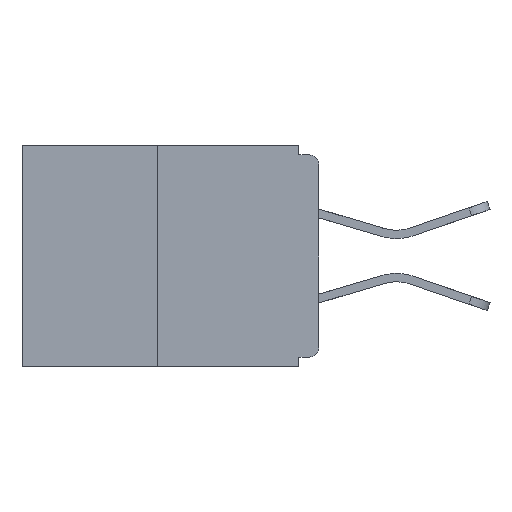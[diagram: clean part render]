
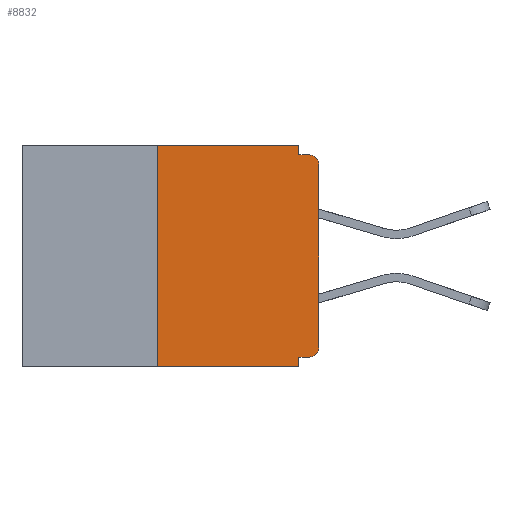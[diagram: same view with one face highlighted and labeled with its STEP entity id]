
A CAD part, left-side view. The second image highlights one B-rep face of the part: STEP entity #8832.
In plain terms, the highlighted planar face has unit normal (-1, 0, 0).
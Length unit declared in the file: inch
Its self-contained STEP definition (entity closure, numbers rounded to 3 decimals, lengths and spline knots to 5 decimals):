
#118 = ORIENTED_EDGE ( 'NONE', *, *, #2227, .F. ) ;
#169 = VERTEX_POINT ( 'NONE', #3268 ) ;
#374 = CARTESIAN_POINT ( 'NONE',  ( 0., 0.031, 0. ) ) ;
#448 = DIRECTION ( 'NONE',  ( 0., -1., 0. ) ) ;
#489 = CARTESIAN_POINT ( 'NONE',  ( 0., 0.46, 0. ) ) ;
#515 = CARTESIAN_POINT ( 'NONE',  ( 0., 0.015, -0.328 ) ) ;
#697 = FACE_OUTER_BOUND ( 'NONE', #9683, .T. ) ;
#770 = CARTESIAN_POINT ( 'NONE',  ( 0., 0., -0.03 ) ) ;
#947 = ORIENTED_EDGE ( 'NONE', *, *, #1244, .T. ) ;
#956 = AXIS2_PLACEMENT_3D ( 'NONE', #5543, #6500, #9940 ) ;
#1126 = CARTESIAN_POINT ( 'NONE',  ( 0., 0., -0.328 ) ) ;
#1204 = DIRECTION ( 'NONE',  ( 0., 1., 0. ) ) ;
#1244 = EDGE_CURVE ( 'NONE', #8211, #8496, #11496, .T. ) ;
#1271 = DIRECTION ( 'NONE',  ( 0., 0., -1. ) ) ;
#1419 = ORIENTED_EDGE ( 'NONE', *, *, #4956, .F. ) ;
#1483 = EDGE_CURVE ( 'NONE', #9737, #9106, #4185, .T. ) ;
#2227 = EDGE_CURVE ( 'NONE', #6264, #7091, #10370, .T. ) ;
#2407 = DIRECTION ( 'NONE',  ( 0., 0., -1. ) ) ;
#2658 = LINE ( 'NONE', #1126, #7680 ) ;
#2899 = CARTESIAN_POINT ( 'NONE',  ( 0., 0., 0. ) ) ;
#2945 = CARTESIAN_POINT ( 'NONE',  ( 0., 0.015, -0.015 ) ) ;
#3024 = VECTOR ( 'NONE', #1271, 39.37008 ) ;
#3134 = VECTOR ( 'NONE', #3990, 39.37008 ) ;
#3176 = AXIS2_PLACEMENT_3D ( 'NONE', #8057, #5354, #6136 ) ;
#3268 = CARTESIAN_POINT ( 'NONE',  ( 0., 0.031, -0.015 ) ) ;
#3499 = DIRECTION ( 'NONE',  ( 0., 0., -1. ) ) ;
#3785 = VECTOR ( 'NONE', #9099, 39.37008 ) ;
#3952 = LINE ( 'NONE', #489, #9489 ) ;
#3979 = CARTESIAN_POINT ( 'NONE',  ( 0., 0.25, 0. ) ) ;
#3990 = DIRECTION ( 'NONE',  ( 0., -1., 0. ) ) ;
#4185 = CIRCLE ( 'NONE', #3176, 0.015 ) ;
#4748 = CARTESIAN_POINT ( 'NONE',  ( 0., 0., -0.015 ) ) ;
#4904 = ORIENTED_EDGE ( 'NONE', *, *, #7840, .F. ) ;
#4956 = EDGE_CURVE ( 'NONE', #10288, #169, #10621, .T. ) ;
#4982 = CARTESIAN_POINT ( 'NONE',  ( 0., 0.46, -0.343 ) ) ;
#5097 = DIRECTION ( 'NONE',  ( -1., 0., 0. ) ) ;
#5354 = DIRECTION ( 'NONE',  ( -1., 0., 0. ) ) ;
#5543 = CARTESIAN_POINT ( 'NONE',  ( 0., 0.46, 0. ) ) ;
#5566 = CARTESIAN_POINT ( 'NONE',  ( 0., 0.031, 0. ) ) ;
#6071 = DIRECTION ( 'NONE',  ( 0., 0., 1. ) ) ;
#6089 = VECTOR ( 'NONE', #6071, 39.37008 ) ;
#6136 = DIRECTION ( 'NONE',  ( 0., 0., -1. ) ) ;
#6165 = EDGE_CURVE ( 'NONE', #169, #9106, #8672, .T. ) ;
#6255 = CARTESIAN_POINT ( 'NONE',  ( 0., 0.031, -0.343 ) ) ;
#6264 = VERTEX_POINT ( 'NONE', #6906 ) ;
#6500 = DIRECTION ( 'NONE',  ( 1., 0., 0. ) ) ;
#6684 = CARTESIAN_POINT ( 'NONE',  ( 0., 0.015, -0.313 ) ) ;
#6906 = CARTESIAN_POINT ( 'NONE',  ( 0., 0.25, -0.343 ) ) ;
#7042 = CARTESIAN_POINT ( 'NONE',  ( 0., 0.25, 0. ) ) ;
#7090 = LINE ( 'NONE', #6255, #9736 ) ;
#7091 = VERTEX_POINT ( 'NONE', #3979 ) ;
#7163 = CARTESIAN_POINT ( 'NONE',  ( 0., 0.031, -0.343 ) ) ;
#7203 = ORIENTED_EDGE ( 'NONE', *, *, #1483, .T. ) ;
#7227 = ORIENTED_EDGE ( 'NONE', *, *, #6165, .F. ) ;
#7264 = ORIENTED_EDGE ( 'NONE', *, *, #7390, .T. ) ;
#7390 = EDGE_CURVE ( 'NONE', #8496, #9737, #11139, .T. ) ;
#7397 = EDGE_CURVE ( 'NONE', #8211, #7767, #2658, .T. ) ;
#7423 = CARTESIAN_POINT ( 'NONE',  ( 0., 0.031, -0.328 ) ) ;
#7680 = VECTOR ( 'NONE', #1204, 39.37008 ) ;
#7767 = VERTEX_POINT ( 'NONE', #7423 ) ;
#7840 = EDGE_CURVE ( 'NONE', #7091, #10288, #3952, .T. ) ;
#7894 = ORIENTED_EDGE ( 'NONE', *, *, #8747, .F. ) ;
#8044 = VERTEX_POINT ( 'NONE', #7163 ) ;
#8057 = CARTESIAN_POINT ( 'NONE',  ( 0., 0.015, -0.03 ) ) ;
#8211 = VERTEX_POINT ( 'NONE', #515 ) ;
#8381 = LINE ( 'NONE', #4982, #11147 ) ;
#8496 = VERTEX_POINT ( 'NONE', #11513 ) ;
#8672 = LINE ( 'NONE', #4748, #3134 ) ;
#8747 = EDGE_CURVE ( 'NONE', #7767, #8044, #7090, .T. ) ;
#8832 = ADVANCED_FACE ( 'NONE', ( #697 ), #9120, .F. ) ;
#9099 = DIRECTION ( 'NONE',  ( 0., 0., 1. ) ) ;
#9106 = VERTEX_POINT ( 'NONE', #2945 ) ;
#9120 = PLANE ( 'NONE',  #956 ) ;
#9489 = VECTOR ( 'NONE', #448, 39.37008 ) ;
#9683 = EDGE_LOOP ( 'NONE', ( #4904, #118, #11397, #7894, #11092, #947, #7264, #7203, #7227, #1419 ) ) ;
#9736 = VECTOR ( 'NONE', #3499, 39.37008 ) ;
#9737 = VERTEX_POINT ( 'NONE', #770 ) ;
#9940 = DIRECTION ( 'NONE',  ( 0., 0., -1. ) ) ;
#10288 = VERTEX_POINT ( 'NONE', #5566 ) ;
#10327 = DIRECTION ( 'NONE',  ( 0., -1., 0. ) ) ;
#10370 = LINE ( 'NONE', #7042, #6089 ) ;
#10507 = EDGE_CURVE ( 'NONE', #6264, #8044, #8381, .T. ) ;
#10621 = LINE ( 'NONE', #374, #3024 ) ;
#11092 = ORIENTED_EDGE ( 'NONE', *, *, #7397, .F. ) ;
#11139 = LINE ( 'NONE', #2899, #3785 ) ;
#11147 = VECTOR ( 'NONE', #10327, 39.37008 ) ;
#11166 = AXIS2_PLACEMENT_3D ( 'NONE', #6684, #5097, #2407 ) ;
#11397 = ORIENTED_EDGE ( 'NONE', *, *, #10507, .T. ) ;
#11496 = CIRCLE ( 'NONE', #11166, 0.015 ) ;
#11513 = CARTESIAN_POINT ( 'NONE',  ( 0., 0., -0.313 ) ) ;
